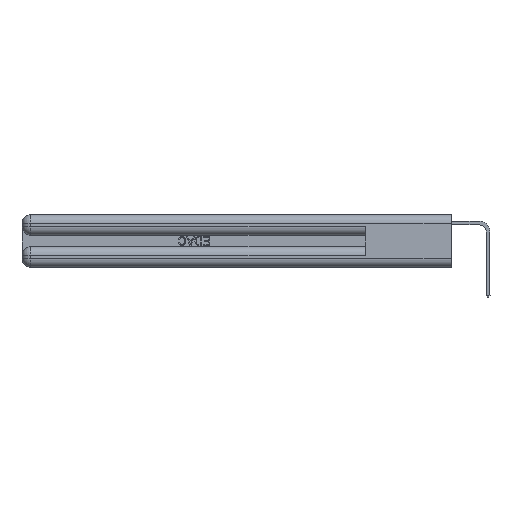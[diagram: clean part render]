
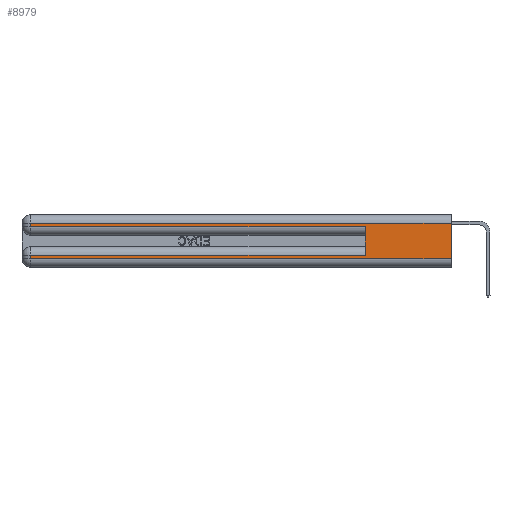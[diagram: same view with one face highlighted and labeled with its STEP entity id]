
A CAD part, left-side view. The second image highlights one B-rep face of the part: STEP entity #8979.
In plain terms, the highlighted planar face has unit normal (-1, 0, 0).
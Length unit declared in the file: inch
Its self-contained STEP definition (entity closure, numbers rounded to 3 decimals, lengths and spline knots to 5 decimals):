
#549 = VECTOR ( 'NONE', #16519, 39.37008 ) ;
#609 = EDGE_CURVE ( 'NONE', #952, #28570, #1854, .T. ) ;
#952 = VERTEX_POINT ( 'NONE', #3590 ) ;
#1098 = ORIENTED_EDGE ( 'NONE', *, *, #22761, .T. ) ;
#1234 = FACE_OUTER_BOUND ( 'NONE', #3420, .T. ) ;
#1514 = CARTESIAN_POINT ( 'NONE',  ( 0., 0., 0.085 ) ) ;
#1526 = CARTESIAN_POINT ( 'NONE',  ( 0., 2.94, 0.285 ) ) ;
#1577 = DIRECTION ( 'NONE',  ( 0., 0., 1. ) ) ;
#1854 = LINE ( 'NONE', #29177, #22270 ) ;
#2950 = ORIENTED_EDGE ( 'NONE', *, *, #24362, .F. ) ;
#3281 = ORIENTED_EDGE ( 'NONE', *, *, #17282, .T. ) ;
#3369 = LINE ( 'NONE', #21601, #8707 ) ;
#3420 = EDGE_LOOP ( 'NONE', ( #9126, #3281, #28557, #3610, #2950, #1098, #16097, #17413 ) ) ;
#3435 = EDGE_CURVE ( 'NONE', #6519, #11568, #22375, .T. ) ;
#3590 = CARTESIAN_POINT ( 'NONE',  ( 0., 0., 0.31 ) ) ;
#3610 = ORIENTED_EDGE ( 'NONE', *, *, #13727, .T. ) ;
#3616 = VECTOR ( 'NONE', #15729, 39.37008 ) ;
#3740 = DIRECTION ( 'NONE',  ( 0., 1., 0. ) ) ;
#3763 = CARTESIAN_POINT ( 'NONE',  ( 0., 0., 0.06 ) ) ;
#4247 = CARTESIAN_POINT ( 'NONE',  ( 0., 2.94, 0.37 ) ) ;
#5591 = EDGE_CURVE ( 'NONE', #12735, #8892, #24624, .T. ) ;
#6519 = VERTEX_POINT ( 'NONE', #25404 ) ;
#6684 = VECTOR ( 'NONE', #12827, 39.37008 ) ;
#8212 = DIRECTION ( 'NONE',  ( 0., 1., 0. ) ) ;
#8512 = CARTESIAN_POINT ( 'NONE',  ( 0., 0., 0.37 ) ) ;
#8707 = VECTOR ( 'NONE', #1577, 39.37008 ) ;
#8892 = VERTEX_POINT ( 'NONE', #1526 ) ;
#8979 = ADVANCED_FACE ( 'NONE', ( #1234 ), #26205, .F. ) ;
#9126 = ORIENTED_EDGE ( 'NONE', *, *, #609, .F. ) ;
#9734 = VECTOR ( 'NONE', #19817, 39.37008 ) ;
#10644 = AXIS2_PLACEMENT_3D ( 'NONE', #8512, #23985, #17547 ) ;
#11431 = CARTESIAN_POINT ( 'NONE',  ( 0., 0., 0.06 ) ) ;
#11568 = VERTEX_POINT ( 'NONE', #21216 ) ;
#12058 = VERTEX_POINT ( 'NONE', #24756 ) ;
#12735 = VERTEX_POINT ( 'NONE', #22302 ) ;
#12827 = DIRECTION ( 'NONE',  ( 0., -1., 0. ) ) ;
#13519 = VERTEX_POINT ( 'NONE', #27279 ) ;
#13727 = EDGE_CURVE ( 'NONE', #8892, #13519, #27321, .T. ) ;
#15135 = VECTOR ( 'NONE', #8212, 39.37008 ) ;
#15729 = DIRECTION ( 'NONE',  ( 0., -1., 0. ) ) ;
#16097 = ORIENTED_EDGE ( 'NONE', *, *, #3435, .T. ) ;
#16519 = DIRECTION ( 'NONE',  ( 0., 0., -1. ) ) ;
#17282 = EDGE_CURVE ( 'NONE', #952, #12735, #24285, .T. ) ;
#17413 = ORIENTED_EDGE ( 'NONE', *, *, #18176, .T. ) ;
#17547 = DIRECTION ( 'NONE',  ( 0., 0., -1. ) ) ;
#18176 = EDGE_CURVE ( 'NONE', #11568, #28570, #24149, .T. ) ;
#19485 = DIRECTION ( 'NONE',  ( 0., 0., -1. ) ) ;
#19817 = DIRECTION ( 'NONE',  ( 0., 0., -1. ) ) ;
#21216 = CARTESIAN_POINT ( 'NONE',  ( 0., 2.94, 0.06 ) ) ;
#21601 = CARTESIAN_POINT ( 'NONE',  ( 0., 0.6, 0.145 ) ) ;
#21848 = CARTESIAN_POINT ( 'NONE',  ( 0., 0., 0.31 ) ) ;
#22270 = VECTOR ( 'NONE', #19485, 39.37008 ) ;
#22302 = CARTESIAN_POINT ( 'NONE',  ( 0., 2.94, 0.31 ) ) ;
#22375 = LINE ( 'NONE', #24192, #9734 ) ;
#22392 = VECTOR ( 'NONE', #3740, 39.37008 ) ;
#22761 = EDGE_CURVE ( 'NONE', #12058, #6519, #28685, .T. ) ;
#23985 = DIRECTION ( 'NONE',  ( 1., 0., 0. ) ) ;
#24149 = LINE ( 'NONE', #3763, #6684 ) ;
#24192 = CARTESIAN_POINT ( 'NONE',  ( 0., 2.94, 0.37 ) ) ;
#24285 = LINE ( 'NONE', #21848, #15135 ) ;
#24362 = EDGE_CURVE ( 'NONE', #12058, #13519, #3369, .T. ) ;
#24624 = LINE ( 'NONE', #4247, #549 ) ;
#24756 = CARTESIAN_POINT ( 'NONE',  ( 0., 0.6, 0.085 ) ) ;
#25404 = CARTESIAN_POINT ( 'NONE',  ( 0., 2.94, 0.085 ) ) ;
#26205 = PLANE ( 'NONE',  #10644 ) ;
#27040 = CARTESIAN_POINT ( 'NONE',  ( 0., 0., 0.285 ) ) ;
#27279 = CARTESIAN_POINT ( 'NONE',  ( 0., 0.6, 0.285 ) ) ;
#27321 = LINE ( 'NONE', #27040, #3616 ) ;
#28557 = ORIENTED_EDGE ( 'NONE', *, *, #5591, .T. ) ;
#28570 = VERTEX_POINT ( 'NONE', #11431 ) ;
#28685 = LINE ( 'NONE', #1514, #22392 ) ;
#29177 = CARTESIAN_POINT ( 'NONE',  ( 0., 0., 0.37 ) ) ;
